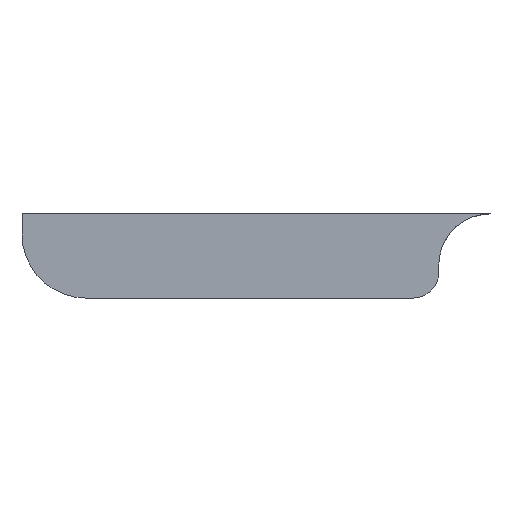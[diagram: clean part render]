
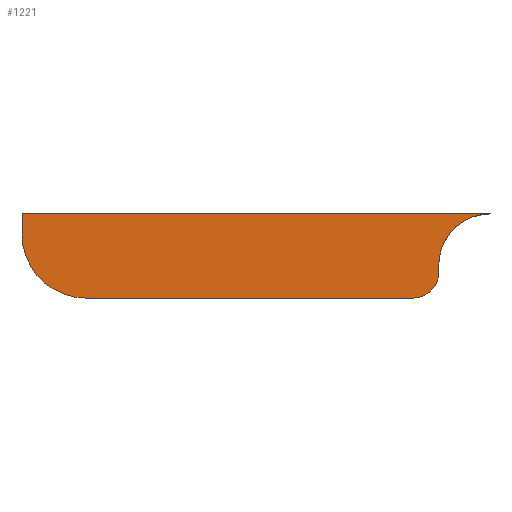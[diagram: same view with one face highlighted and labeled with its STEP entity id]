
A CAD part, left-side view. The second image highlights one B-rep face of the part: STEP entity #1221.
In plain terms, the highlighted planar face has unit normal (-1, 0, 0).
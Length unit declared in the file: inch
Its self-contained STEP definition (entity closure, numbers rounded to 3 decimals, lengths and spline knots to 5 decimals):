
#4 = VERTEX_POINT ( 'NONE', #1191 ) ;
#13 = VECTOR ( 'NONE', #1011, 39.37008 ) ;
#30 = VERTEX_POINT ( 'NONE', #538 ) ;
#57 = CARTESIAN_POINT ( 'NONE',  ( 8.2556, -0.71157, -0.53412 ) ) ;
#75 = AXIS2_PLACEMENT_3D ( 'NONE', #585, #593, #1238 ) ;
#80 = CARTESIAN_POINT ( 'NONE',  ( 8.2556, -1.79442, -0.62992 ) ) ;
#81 = ORIENTED_EDGE ( 'NONE', *, *, #512, .T. ) ;
#123 = LINE ( 'NONE', #537, #1081 ) ;
#137 = FACE_OUTER_BOUND ( 'NONE', #996, .T. ) ;
#158 = DIRECTION ( 'NONE',  ( 0., 1., 0. ) ) ;
#180 = VERTEX_POINT ( 'NONE', #262 ) ;
#198 = VERTEX_POINT ( 'NONE', #80 ) ;
#217 = VECTOR ( 'NONE', #660, 39.37008 ) ;
#222 = VERTEX_POINT ( 'NONE', #718 ) ;
#241 = DIRECTION ( 'NONE',  ( 0., 0., 1. ) ) ;
#244 = CARTESIAN_POINT ( 'NONE',  ( 8.2556, -1.79442, -1.11943 ) ) ;
#262 = CARTESIAN_POINT ( 'NONE',  ( 8.2556, -0.71157, -0.73097 ) ) ;
#327 = CARTESIAN_POINT ( 'NONE',  ( 8.2556, -1.79442, -0.65223 ) ) ;
#392 = AXIS2_PLACEMENT_3D ( 'NONE', #1120, #556, #1203 ) ;
#406 = AXIS2_PLACEMENT_3D ( 'NONE', #445, #1113, #548 ) ;
#431 = VERTEX_POINT ( 'NONE', #991 ) ;
#445 = CARTESIAN_POINT ( 'NONE',  ( 8.2556, -1.71568, -0.65223 ) ) ;
#454 = AXIS2_PLACEMENT_3D ( 'NONE', #57, #762, #158 ) ;
#473 = ORIENTED_EDGE ( 'NONE', *, *, #644, .F. ) ;
#485 = PLANE ( 'NONE',  #75 ) ;
#493 = EDGE_CURVE ( 'NONE', #198, #994, #540, .T. ) ;
#496 = ORIENTED_EDGE ( 'NONE', *, *, #624, .F. ) ;
#511 = EDGE_CURVE ( 'NONE', #431, #994, #980, .T. ) ;
#512 = EDGE_CURVE ( 'NONE', #222, #180, #791, .T. ) ;
#523 = EDGE_CURVE ( 'NONE', #431, #180, #1236, .T. ) ;
#533 = EDGE_CURVE ( 'NONE', #30, #198, #755, .T. ) ;
#537 = CARTESIAN_POINT ( 'NONE',  ( 8.2556, -0.51472, -0.70907 ) ) ;
#538 = CARTESIAN_POINT ( 'NONE',  ( 8.2556, -1.9519, -0.47244 ) ) ;
#540 = LINE ( 'NONE', #244, #13 ) ;
#548 = DIRECTION ( 'NONE',  ( 0., 1., 0. ) ) ;
#556 = DIRECTION ( 'NONE',  ( -1., 0., 0. ) ) ;
#575 = ORIENTED_EDGE ( 'NONE', *, *, #533, .F. ) ;
#585 = CARTESIAN_POINT ( 'NONE',  ( 8.2556, -5.33922, 2.87623 ) ) ;
#593 = DIRECTION ( 'NONE',  ( 1., 0., 0. ) ) ;
#603 = ORIENTED_EDGE ( 'NONE', *, *, #493, .F. ) ;
#624 = EDGE_CURVE ( 'NONE', #4, #30, #1152, .T. ) ;
#644 = EDGE_CURVE ( 'NONE', #222, #4, #123, .T. ) ;
#660 = DIRECTION ( 'NONE',  ( 0., 1., 0. ) ) ;
#715 = ORIENTED_EDGE ( 'NONE', *, *, #511, .T. ) ;
#718 = CARTESIAN_POINT ( 'NONE',  ( 8.2556, -0.51472, -0.53412 ) ) ;
#755 = CIRCLE ( 'NONE', #392, 0.15748 ) ;
#762 = DIRECTION ( 'NONE',  ( -1., 0., 0. ) ) ;
#791 = CIRCLE ( 'NONE', #454, 0.19685 ) ;
#920 = DIRECTION ( 'NONE',  ( 0., -1., 0. ) ) ;
#980 = CIRCLE ( 'NONE', #406, 0.07874 ) ;
#991 = CARTESIAN_POINT ( 'NONE',  ( 8.2556, -1.71568, -0.73097 ) ) ;
#994 = VERTEX_POINT ( 'NONE', #327 ) ;
#996 = EDGE_LOOP ( 'NONE', ( #81, #1186, #715, #603, #575, #496, #473 ) ) ;
#1011 = DIRECTION ( 'NONE',  ( 0., 0., -1. ) ) ;
#1081 = VECTOR ( 'NONE', #241, 39.37008 ) ;
#1113 = DIRECTION ( 'NONE',  ( -1., 0., 0. ) ) ;
#1119 = VECTOR ( 'NONE', #920, 39.37008 ) ;
#1120 = CARTESIAN_POINT ( 'NONE',  ( 8.2556, -1.9519, -0.62992 ) ) ;
#1152 = LINE ( 'NONE', #1184, #1119 ) ;
#1184 = CARTESIAN_POINT ( 'NONE',  ( 8.2556, 1.32551, -0.47244 ) ) ;
#1186 = ORIENTED_EDGE ( 'NONE', *, *, #523, .F. ) ;
#1191 = CARTESIAN_POINT ( 'NONE',  ( 8.2556, -0.51472, -0.47244 ) ) ;
#1198 = CARTESIAN_POINT ( 'NONE',  ( 8.2556, -0.47716, -0.73097 ) ) ;
#1203 = DIRECTION ( 'NONE',  ( 0., 1., 0. ) ) ;
#1221 = ADVANCED_FACE ( 'NONE', ( #137 ), #485, .F. ) ;
#1236 = LINE ( 'NONE', #1198, #217 ) ;
#1238 = DIRECTION ( 'NONE',  ( 0., 1., 0. ) ) ;
